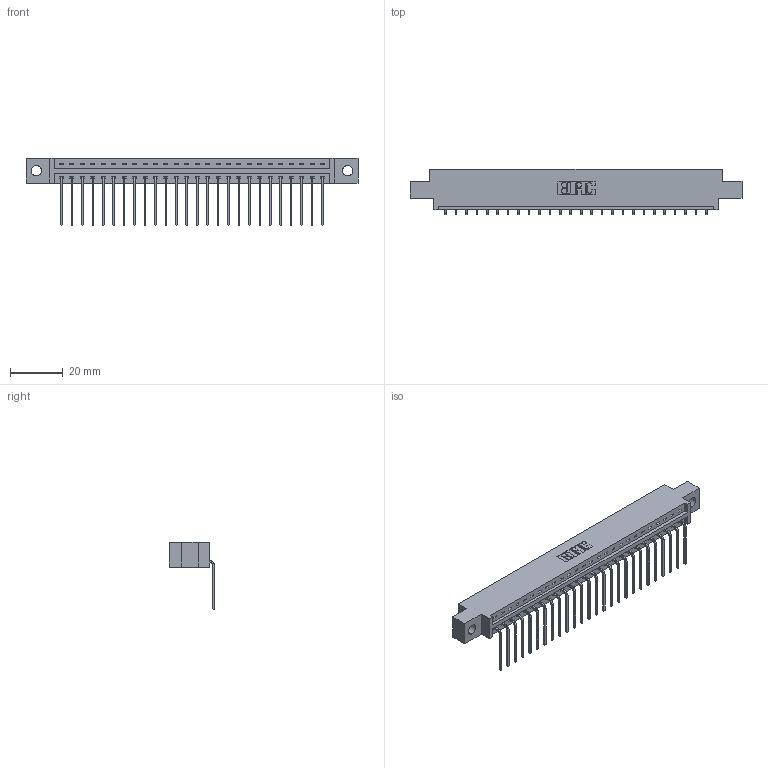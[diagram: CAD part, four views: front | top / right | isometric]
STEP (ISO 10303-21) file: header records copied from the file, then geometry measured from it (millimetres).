
FILE_DESCRIPTION (( 'STEP AP203' ), '1' );
FILE_NAME ('387-026-559-604.STEP', '2018-09-16T12:10:22', ( '' ), ( '' ), 'SwSTEP 2.0', 'SolidWorks 2016', '' );
FILE_SCHEMA (( 'CONFIG_CONTROL_DESIGN' ));
Length unit declared in the file: inch
Products named in the file (3): 345-292-001_558 559 Tail - 1; 387-026-559-604; 337 Part_0.170 Offset - 0.156 Dia-TH
Assembly tree (27 placements, depth 2):
  387-026-559-604
    337 Part_0.170 Offset - 0.156 Dia-TH
    345-292-001_558 559 Tail - 1  x26
Bounding box: 126.03 x 17.09 x 25.53 mm (x, y, z)
Volume: 12780.2 mm3; surface area: 13541.6 mm2
Topology: 27 solids, 27 shells, 1782 faces, 5367 edges, 3542 vertices
Faces by surface type: plane 1322, cylinder 460
Entity records: 21615 total; most frequent: CARTESIAN_POINT 3772, ORIENTED_EDGE 3734, DIRECTION 3207, EDGE_CURVE 1867, LINE 1739, VECTOR 1739, VERTEX_POINT 1242, AXIS2_PLACEMENT_3D 734
